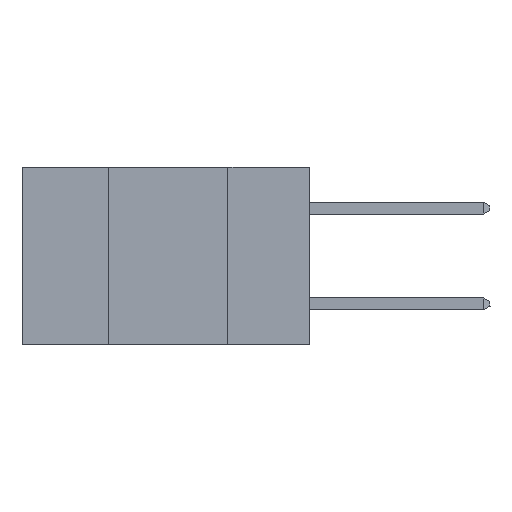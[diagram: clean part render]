
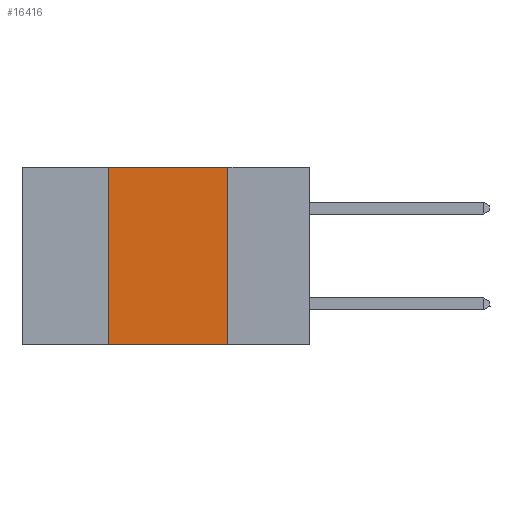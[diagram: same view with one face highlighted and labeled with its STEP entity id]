
A CAD part, left-side view. The second image highlights one B-rep face of the part: STEP entity #16416.
In plain terms, the highlighted planar face has unit normal (-1, 0, 0).
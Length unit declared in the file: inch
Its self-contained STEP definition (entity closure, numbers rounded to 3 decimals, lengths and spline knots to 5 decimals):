
#1486 = CARTESIAN_POINT ( 'NONE',  ( 0., 0.17, 0. ) ) ;
#2127 = LINE ( 'NONE', #32841, #18220 ) ;
#2538 = EDGE_LOOP ( 'NONE', ( #24683, #11686, #4341, #13718 ) ) ;
#4341 = ORIENTED_EDGE ( 'NONE', *, *, #33301, .F. ) ;
#7550 = DIRECTION ( 'NONE',  ( 1., 0., 0. ) ) ;
#8096 = CARTESIAN_POINT ( 'NONE',  ( 0., 0.42, 0. ) ) ;
#8273 = DIRECTION ( 'NONE',  ( 0., 0., 1. ) ) ;
#10417 = PLANE ( 'NONE',  #18637 ) ;
#11686 = ORIENTED_EDGE ( 'NONE', *, *, #16499, .F. ) ;
#12570 = VERTEX_POINT ( 'NONE', #14350 ) ;
#12764 = LINE ( 'NONE', #13114, #20158 ) ;
#13114 = CARTESIAN_POINT ( 'NONE',  ( 0., 0.6, 0. ) ) ;
#13718 = ORIENTED_EDGE ( 'NONE', *, *, #28152, .T. ) ;
#14182 = VECTOR ( 'NONE', #21683, 39.37008 ) ;
#14350 = CARTESIAN_POINT ( 'NONE',  ( 0., 0.17, -0.37 ) ) ;
#15299 = DIRECTION ( 'NONE',  ( 0., 0., -1. ) ) ;
#16119 = VECTOR ( 'NONE', #8273, 39.37008 ) ;
#16416 = ADVANCED_FACE ( 'NONE', ( #33768 ), #10417, .F. ) ;
#16499 = EDGE_CURVE ( 'NONE', #25705, #25975, #12764, .T. ) ;
#18220 = VECTOR ( 'NONE', #21740, 39.37008 ) ;
#18637 = AXIS2_PLACEMENT_3D ( 'NONE', #35035, #7550, #15299 ) ;
#20158 = VECTOR ( 'NONE', #26771, 39.37008 ) ;
#21433 = VERTEX_POINT ( 'NONE', #34017 ) ;
#21495 = LINE ( 'NONE', #32426, #14182 ) ;
#21683 = DIRECTION ( 'NONE',  ( 0., 0., -1. ) ) ;
#21740 = DIRECTION ( 'NONE',  ( 0., -1., 0. ) ) ;
#24368 = CARTESIAN_POINT ( 'NONE',  ( 0., 0.42, 0. ) ) ;
#24683 = ORIENTED_EDGE ( 'NONE', *, *, #25724, .F. ) ;
#25705 = VERTEX_POINT ( 'NONE', #24368 ) ;
#25724 = EDGE_CURVE ( 'NONE', #25975, #12570, #21495, .T. ) ;
#25975 = VERTEX_POINT ( 'NONE', #1486 ) ;
#26771 = DIRECTION ( 'NONE',  ( 0., -1., 0. ) ) ;
#26962 = LINE ( 'NONE', #8096, #16119 ) ;
#28152 = EDGE_CURVE ( 'NONE', #21433, #12570, #2127, .T. ) ;
#32426 = CARTESIAN_POINT ( 'NONE',  ( 0., 0.17, 0. ) ) ;
#32841 = CARTESIAN_POINT ( 'NONE',  ( 0., 0.6, -0.37 ) ) ;
#33301 = EDGE_CURVE ( 'NONE', #21433, #25705, #26962, .T. ) ;
#33768 = FACE_OUTER_BOUND ( 'NONE', #2538, .T. ) ;
#34017 = CARTESIAN_POINT ( 'NONE',  ( 0., 0.42, -0.37 ) ) ;
#35035 = CARTESIAN_POINT ( 'NONE',  ( 0., 0.6, 0. ) ) ;
